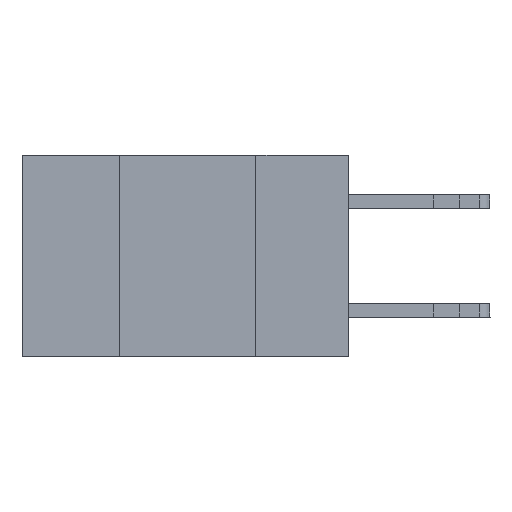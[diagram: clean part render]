
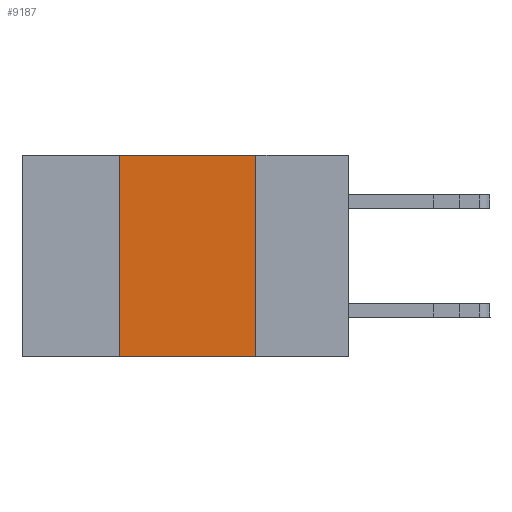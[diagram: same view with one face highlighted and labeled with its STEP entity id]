
A CAD part, left-side view. The second image highlights one B-rep face of the part: STEP entity #9187.
In plain terms, the highlighted planar face has unit normal (-1, 0, 0).
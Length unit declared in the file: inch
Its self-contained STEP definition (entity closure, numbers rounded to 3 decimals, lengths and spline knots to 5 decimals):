
#1280 = EDGE_CURVE ( 'NONE', #14454, #6692, #19788, .T. ) ;
#1381 = EDGE_CURVE ( 'NONE', #4951, #14454, #18532, .T. ) ;
#1779 = ORIENTED_EDGE ( 'NONE', *, *, #1381, .F. ) ;
#3277 = ORIENTED_EDGE ( 'NONE', *, *, #1280, .F. ) ;
#3377 = VECTOR ( 'NONE', #12949, 39.37008 ) ;
#3932 = CARTESIAN_POINT ( 'NONE',  ( 0., 0.17, -0.37 ) ) ;
#4855 = CARTESIAN_POINT ( 'NONE',  ( 0., 0.6, 0. ) ) ;
#4951 = VERTEX_POINT ( 'NONE', #17596 ) ;
#5311 = VECTOR ( 'NONE', #12062, 39.37008 ) ;
#5939 = EDGE_CURVE ( 'NONE', #6692, #12147, #11673, .T. ) ;
#6692 = VERTEX_POINT ( 'NONE', #8467 ) ;
#8317 = EDGE_LOOP ( 'NONE', ( #18847, #3277, #1779, #8722 ) ) ;
#8352 = CARTESIAN_POINT ( 'NONE',  ( 0., 0.6, 0. ) ) ;
#8467 = CARTESIAN_POINT ( 'NONE',  ( 0., 0.17, 0. ) ) ;
#8722 = ORIENTED_EDGE ( 'NONE', *, *, #12245, .T. ) ;
#9116 = DIRECTION ( 'NONE',  ( 0., 0., 1. ) ) ;
#9187 = ADVANCED_FACE ( 'NONE', ( #19226 ), #20266, .F. ) ;
#9240 = DIRECTION ( 'NONE',  ( 1., 0., 0. ) ) ;
#9779 = CARTESIAN_POINT ( 'NONE',  ( 0., 0.17, 0. ) ) ;
#10393 = CARTESIAN_POINT ( 'NONE',  ( 0., 0.42, 0. ) ) ;
#10871 = VECTOR ( 'NONE', #17738, 39.37008 ) ;
#11673 = LINE ( 'NONE', #9779, #3377 ) ;
#11865 = AXIS2_PLACEMENT_3D ( 'NONE', #4855, #9240, #12398 ) ;
#12062 = DIRECTION ( 'NONE',  ( 0., -1., 0. ) ) ;
#12147 = VERTEX_POINT ( 'NONE', #3932 ) ;
#12245 = EDGE_CURVE ( 'NONE', #4951, #12147, #20120, .T. ) ;
#12398 = DIRECTION ( 'NONE',  ( 0., 0., -1. ) ) ;
#12949 = DIRECTION ( 'NONE',  ( 0., 0., -1. ) ) ;
#14339 = VECTOR ( 'NONE', #9116, 39.37008 ) ;
#14454 = VERTEX_POINT ( 'NONE', #17966 ) ;
#15200 = CARTESIAN_POINT ( 'NONE',  ( 0., 0.6, -0.37 ) ) ;
#17596 = CARTESIAN_POINT ( 'NONE',  ( 0., 0.42, -0.37 ) ) ;
#17738 = DIRECTION ( 'NONE',  ( 0., -1., 0. ) ) ;
#17966 = CARTESIAN_POINT ( 'NONE',  ( 0., 0.42, 0. ) ) ;
#18532 = LINE ( 'NONE', #10393, #14339 ) ;
#18847 = ORIENTED_EDGE ( 'NONE', *, *, #5939, .F. ) ;
#19226 = FACE_OUTER_BOUND ( 'NONE', #8317, .T. ) ;
#19788 = LINE ( 'NONE', #8352, #10871 ) ;
#20120 = LINE ( 'NONE', #15200, #5311 ) ;
#20266 = PLANE ( 'NONE',  #11865 ) ;
